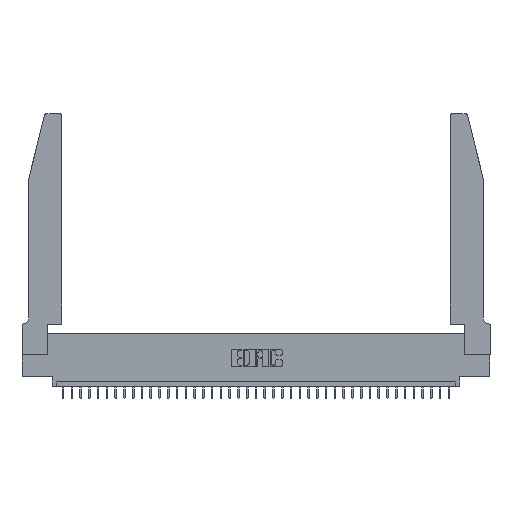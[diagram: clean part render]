
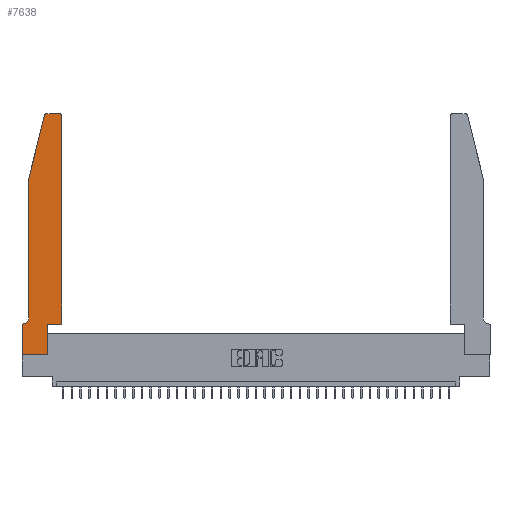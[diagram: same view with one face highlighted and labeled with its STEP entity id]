
A CAD part, top view. The second image highlights one B-rep face of the part: STEP entity #7638.
In plain terms, the highlighted planar face has unit normal (0, 0, 1).
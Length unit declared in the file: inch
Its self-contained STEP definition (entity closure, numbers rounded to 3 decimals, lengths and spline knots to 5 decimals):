
#880 = EDGE_CURVE ( 'NONE', #3457, #3141, #18822, .T. ) ;
#958 = VERTEX_POINT ( 'NONE', #10893 ) ;
#1568 = LINE ( 'NONE', #13405, #18567 ) ;
#2152 = DIRECTION ( 'NONE',  ( -0.239, -0.971, 0. ) ) ;
#2162 = EDGE_LOOP ( 'NONE', ( #15494, #14746, #32928, #2841, #24951, #36741, #26745, #30725, #31892, #13840, #21413, #18317 ) ) ;
#2381 = CARTESIAN_POINT ( 'NONE',  ( 0.2605, 2.75, 0.37 ) ) ;
#2841 = ORIENTED_EDGE ( 'NONE', *, *, #37252, .T. ) ;
#3141 = VERTEX_POINT ( 'NONE', #25985 ) ;
#3457 = VERTEX_POINT ( 'NONE', #20050 ) ;
#3861 = EDGE_CURVE ( 'NONE', #17282, #8394, #19427, .T. ) ;
#4676 = DIRECTION ( 'NONE',  ( 0., 1., 0. ) ) ;
#4809 = DIRECTION ( 'NONE',  ( 1., 0., 0. ) ) ;
#4860 = VERTEX_POINT ( 'NONE', #20299 ) ;
#4997 = CARTESIAN_POINT ( 'NONE',  ( 0.4205, 2.72, 0.37 ) ) ;
#5402 = CARTESIAN_POINT ( 'NONE',  ( 0.284, 2.72, 0.37 ) ) ;
#5480 = CARTESIAN_POINT ( 'NONE',  ( 0.2865, 0.35, 0.37 ) ) ;
#5579 = CARTESIAN_POINT ( 'NONE',  ( 0.4505, 0.35, 0.37 ) ) ;
#5831 = CARTESIAN_POINT ( 'NONE',  ( 0., 0., 0.37 ) ) ;
#6254 = VECTOR ( 'NONE', #20306, 39.37008 ) ;
#6381 = EDGE_CURVE ( 'NONE', #19194, #4860, #23908, .T. ) ;
#7034 = DIRECTION ( 'NONE',  ( 1., 0., 0. ) ) ;
#7336 = PLANE ( 'NONE',  #37031 ) ;
#7638 = ADVANCED_FACE ( 'NONE', ( #27942 ), #7336, .T. ) ;
#7766 = CARTESIAN_POINT ( 'NONE',  ( 0., 0.35, 0.37 ) ) ;
#8010 = CARTESIAN_POINT ( 'NONE',  ( 0.0755, 2., 0.37 ) ) ;
#8358 = LINE ( 'NONE', #5831, #28354 ) ;
#8394 = VERTEX_POINT ( 'NONE', #19092 ) ;
#8455 = VECTOR ( 'NONE', #34018, 39.37008 ) ;
#9278 = CARTESIAN_POINT ( 'NONE',  ( 0.0755, 2., 0.37 ) ) ;
#10696 = CARTESIAN_POINT ( 'NONE',  ( 0.4505, 0.35, 0.37 ) ) ;
#10820 = CARTESIAN_POINT ( 'NONE',  ( 0.2865, 0.35, 0.37 ) ) ;
#10857 = CARTESIAN_POINT ( 'NONE',  ( 0., 0., 0.37 ) ) ;
#10893 = CARTESIAN_POINT ( 'NONE',  ( 0.0055, 0.35, 0.37 ) ) ;
#11105 = VECTOR ( 'NONE', #2152, 39.37008 ) ;
#11194 = DIRECTION ( 'NONE',  ( 0., 0., 1. ) ) ;
#11655 = VECTOR ( 'NONE', #35810, 39.37008 ) ;
#13069 = EDGE_CURVE ( 'NONE', #3141, #18718, #31885, .T. ) ;
#13166 = DIRECTION ( 'NONE',  ( 0., 1., 0. ) ) ;
#13183 = EDGE_CURVE ( 'NONE', #37804, #19194, #1568, .T. ) ;
#13405 = CARTESIAN_POINT ( 'NONE',  ( 0.4505, 0.35, 0.37 ) ) ;
#13840 = ORIENTED_EDGE ( 'NONE', *, *, #25443, .T. ) ;
#13948 = DIRECTION ( 'NONE',  ( 1., 0., 0. ) ) ;
#14312 = CARTESIAN_POINT ( 'NONE',  ( 0., 0.35, 0.37 ) ) ;
#14746 = ORIENTED_EDGE ( 'NONE', *, *, #880, .T. ) ;
#15494 = ORIENTED_EDGE ( 'NONE', *, *, #19351, .T. ) ;
#15573 = AXIS2_PLACEMENT_3D ( 'NONE', #29881, #21295, #33156 ) ;
#17282 = VERTEX_POINT ( 'NONE', #7766 ) ;
#17315 = LINE ( 'NONE', #8010, #20976 ) ;
#17523 = LINE ( 'NONE', #2381, #11655 ) ;
#18317 = ORIENTED_EDGE ( 'NONE', *, *, #6381, .T. ) ;
#18567 = VECTOR ( 'NONE', #4676, 39.37008 ) ;
#18718 = VERTEX_POINT ( 'NONE', #9278 ) ;
#18822 = CIRCLE ( 'NONE', #27523, 0.03 ) ;
#19092 = CARTESIAN_POINT ( 'NONE',  ( 0., 0., 0.37 ) ) ;
#19194 = VERTEX_POINT ( 'NONE', #36818 ) ;
#19351 = EDGE_CURVE ( 'NONE', #4860, #3457, #17523, .T. ) ;
#19376 = VERTEX_POINT ( 'NONE', #5480 ) ;
#19427 = LINE ( 'NONE', #10857, #8455 ) ;
#20050 = CARTESIAN_POINT ( 'NONE',  ( 0.284, 2.75, 0.37 ) ) ;
#20111 = CARTESIAN_POINT ( 'NONE',  ( 0.0755, 0.35, 0.37 ) ) ;
#20121 = EDGE_CURVE ( 'NONE', #26919, #19376, #25611, .T. ) ;
#20214 = DIRECTION ( 'NONE',  ( 1., 0., 0. ) ) ;
#20299 = CARTESIAN_POINT ( 'NONE',  ( 0.4205, 2.75, 0.37 ) ) ;
#20306 = DIRECTION ( 'NONE',  ( -1., 0., 0. ) ) ;
#20976 = VECTOR ( 'NONE', #37961, 39.37008 ) ;
#21295 = DIRECTION ( 'NONE',  ( 0., 0., -1. ) ) ;
#21413 = ORIENTED_EDGE ( 'NONE', *, *, #13183, .T. ) ;
#21744 = CARTESIAN_POINT ( 'NONE',  ( 0.0755, 0.42, 0.37 ) ) ;
#22386 = EDGE_CURVE ( 'NONE', #34535, #958, #32354, .T. ) ;
#23463 = DIRECTION ( 'NONE',  ( 1., 0., 0. ) ) ;
#23908 = CIRCLE ( 'NONE', #31372, 0.03 ) ;
#23976 = EDGE_CURVE ( 'NONE', #958, #17282, #34921, .T. ) ;
#24295 = CARTESIAN_POINT ( 'NONE',  ( 0.2865, 0., 0.37 ) ) ;
#24951 = ORIENTED_EDGE ( 'NONE', *, *, #22386, .T. ) ;
#25082 = LINE ( 'NONE', #10696, #34300 ) ;
#25443 = EDGE_CURVE ( 'NONE', #19376, #37804, #25082, .T. ) ;
#25605 = DIRECTION ( 'NONE',  ( 0., 0., 1. ) ) ;
#25611 = LINE ( 'NONE', #10820, #32836 ) ;
#25624 = DIRECTION ( 'NONE',  ( 0., 0., 1. ) ) ;
#25985 = CARTESIAN_POINT ( 'NONE',  ( 0.25487, 2.72718, 0.37 ) ) ;
#26745 = ORIENTED_EDGE ( 'NONE', *, *, #3861, .T. ) ;
#26919 = VERTEX_POINT ( 'NONE', #24295 ) ;
#27523 = AXIS2_PLACEMENT_3D ( 'NONE', #5402, #25624, #13948 ) ;
#27942 = FACE_OUTER_BOUND ( 'NONE', #2162, .T. ) ;
#28354 = VECTOR ( 'NONE', #20214, 39.37008 ) ;
#29881 = CARTESIAN_POINT ( 'NONE',  ( 0.0055, 0.42, 0.37 ) ) ;
#30725 = ORIENTED_EDGE ( 'NONE', *, *, #34420, .T. ) ;
#31372 = AXIS2_PLACEMENT_3D ( 'NONE', #4997, #11194, #4809 ) ;
#31885 = LINE ( 'NONE', #34230, #11105 ) ;
#31892 = ORIENTED_EDGE ( 'NONE', *, *, #20121, .T. ) ;
#32354 = CIRCLE ( 'NONE', #15573, 0.07 ) ;
#32836 = VECTOR ( 'NONE', #13166, 39.37008 ) ;
#32928 = ORIENTED_EDGE ( 'NONE', *, *, #13069, .T. ) ;
#33156 = DIRECTION ( 'NONE',  ( -1., 0., 0. ) ) ;
#34018 = DIRECTION ( 'NONE',  ( 0., -1., 0. ) ) ;
#34230 = CARTESIAN_POINT ( 'NONE',  ( 0.0755, 2., 0.37 ) ) ;
#34300 = VECTOR ( 'NONE', #7034, 39.37008 ) ;
#34420 = EDGE_CURVE ( 'NONE', #8394, #26919, #8358, .T. ) ;
#34535 = VERTEX_POINT ( 'NONE', #21744 ) ;
#34921 = LINE ( 'NONE', #20111, #6254 ) ;
#35810 = DIRECTION ( 'NONE',  ( -1., 0., 0. ) ) ;
#36741 = ORIENTED_EDGE ( 'NONE', *, *, #23976, .T. ) ;
#36818 = CARTESIAN_POINT ( 'NONE',  ( 0.4505, 2.72, 0.37 ) ) ;
#37031 = AXIS2_PLACEMENT_3D ( 'NONE', #14312, #25605, #23463 ) ;
#37252 = EDGE_CURVE ( 'NONE', #18718, #34535, #17315, .T. ) ;
#37804 = VERTEX_POINT ( 'NONE', #5579 ) ;
#37961 = DIRECTION ( 'NONE',  ( 0., -1., 0. ) ) ;
